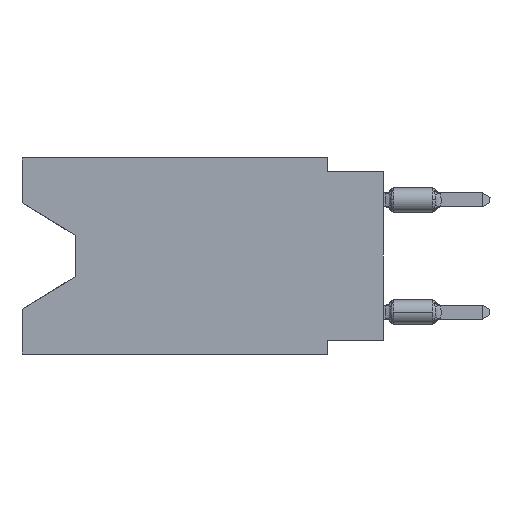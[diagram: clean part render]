
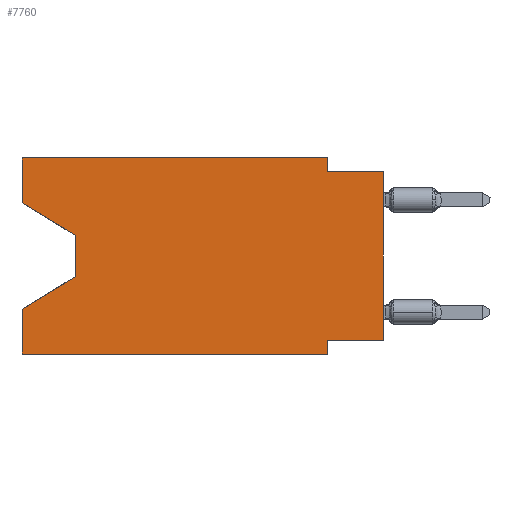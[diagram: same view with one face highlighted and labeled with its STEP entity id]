
A CAD part, left-side view. The second image highlights one B-rep face of the part: STEP entity #7760.
In plain terms, the highlighted planar face has unit normal (-1, 0, 0).
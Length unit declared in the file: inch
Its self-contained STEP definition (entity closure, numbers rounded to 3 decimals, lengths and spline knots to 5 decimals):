
#318 = DIRECTION ( 'NONE',  ( 0., -1., 0. ) ) ;
#1150 = VECTOR ( 'NONE', #9499, 39.37008 ) ;
#1841 = VECTOR ( 'NONE', #16102, 39.37008 ) ;
#2017 = VECTOR ( 'NONE', #31984, 39.37008 ) ;
#2432 = LINE ( 'NONE', #25437, #11160 ) ;
#2998 = LINE ( 'NONE', #15997, #26203 ) ;
#3297 = CARTESIAN_POINT ( 'NONE',  ( 0., 0.645, -0.08025 ) ) ;
#4237 = ORIENTED_EDGE ( 'NONE', *, *, #34123, .F. ) ;
#4421 = LINE ( 'NONE', #14240, #36159 ) ;
#4479 = EDGE_CURVE ( 'NONE', #39658, #11917, #41431, .T. ) ;
#4658 = EDGE_CURVE ( 'NONE', #16934, #17567, #22708, .T. ) ;
#4976 = DIRECTION ( 'NONE',  ( 0., -1., 0. ) ) ;
#7413 = EDGE_CURVE ( 'NONE', #12350, #29813, #33748, .T. ) ;
#7518 = VERTEX_POINT ( 'NONE', #34410 ) ;
#7760 = ADVANCED_FACE ( 'NONE', ( #36956 ), #10735, .F. ) ;
#8228 = VECTOR ( 'NONE', #39567, 39.37008 ) ;
#8532 = VECTOR ( 'NONE', #36527, 39.37008 ) ;
#9341 = CARTESIAN_POINT ( 'NONE',  ( 0., 0., -0.025 ) ) ;
#9465 = CARTESIAN_POINT ( 'NONE',  ( 0., 0.55, -0.138 ) ) ;
#9499 = DIRECTION ( 'NONE',  ( 0., -0.855, -0.519 ) ) ;
#10164 = ORIENTED_EDGE ( 'NONE', *, *, #4479, .F. ) ;
#10735 = PLANE ( 'NONE',  #25814 ) ;
#11044 = VERTEX_POINT ( 'NONE', #17117 ) ;
#11150 = DIRECTION ( 'NONE',  ( 1., 0., 0. ) ) ;
#11160 = VECTOR ( 'NONE', #28229, 39.37008 ) ;
#11300 = ORIENTED_EDGE ( 'NONE', *, *, #36646, .F. ) ;
#11349 = DIRECTION ( 'NONE',  ( 0., 0., -1. ) ) ;
#11610 = VECTOR ( 'NONE', #28250, 39.37008 ) ;
#11917 = VERTEX_POINT ( 'NONE', #25772 ) ;
#12350 = VERTEX_POINT ( 'NONE', #20180 ) ;
#12789 = EDGE_CURVE ( 'NONE', #12350, #17078, #19299, .T. ) ;
#13337 = EDGE_LOOP ( 'NONE', ( #37701, #33000, #29234, #34157, #21272, #28430, #10164, #22071, #40566, #4237, #11300, #14160 ) ) ;
#13786 = LINE ( 'NONE', #23162, #8228 ) ;
#14160 = ORIENTED_EDGE ( 'NONE', *, *, #7413, .F. ) ;
#14240 = CARTESIAN_POINT ( 'NONE',  ( 0., 0., 0. ) ) ;
#14270 = EDGE_CURVE ( 'NONE', #26141, #36155, #41878, .T. ) ;
#14952 = CARTESIAN_POINT ( 'NONE',  ( 0., 0.1, -0.025 ) ) ;
#15997 = CARTESIAN_POINT ( 'NONE',  ( 0., 0.645, -0.35 ) ) ;
#16000 = CARTESIAN_POINT ( 'NONE',  ( 0., 0.55, -0.138 ) ) ;
#16102 = DIRECTION ( 'NONE',  ( 0., 0., 1. ) ) ;
#16518 = VERTEX_POINT ( 'NONE', #24857 ) ;
#16934 = VERTEX_POINT ( 'NONE', #14952 ) ;
#17078 = VERTEX_POINT ( 'NONE', #16000 ) ;
#17117 = CARTESIAN_POINT ( 'NONE',  ( 0., 0.55, -0.212 ) ) ;
#17206 = CARTESIAN_POINT ( 'NONE',  ( 0., 0.645, -0.26975 ) ) ;
#17561 = CARTESIAN_POINT ( 'NONE',  ( 0., 0.645, 0. ) ) ;
#17567 = VERTEX_POINT ( 'NONE', #9341 ) ;
#17666 = CARTESIAN_POINT ( 'NONE',  ( 0., 0.645, -0.35 ) ) ;
#18303 = EDGE_CURVE ( 'NONE', #26141, #7518, #2998, .T. ) ;
#18371 = VECTOR ( 'NONE', #4976, 39.37008 ) ;
#19299 = LINE ( 'NONE', #3297, #1150 ) ;
#19459 = DIRECTION ( 'NONE',  ( 0., 0., -1. ) ) ;
#20180 = CARTESIAN_POINT ( 'NONE',  ( 0., 0.645, -0.08025 ) ) ;
#21272 = ORIENTED_EDGE ( 'NONE', *, *, #18303, .T. ) ;
#22071 = ORIENTED_EDGE ( 'NONE', *, *, #28123, .T. ) ;
#22308 = CARTESIAN_POINT ( 'NONE',  ( 0., 0.645, 0. ) ) ;
#22396 = CARTESIAN_POINT ( 'NONE',  ( 0., 0.1, -0.35 ) ) ;
#22708 = LINE ( 'NONE', #28886, #28621 ) ;
#23162 = CARTESIAN_POINT ( 'NONE',  ( 0., 0.55, -0.212 ) ) ;
#24857 = CARTESIAN_POINT ( 'NONE',  ( 0., 0.1, 0. ) ) ;
#25437 = CARTESIAN_POINT ( 'NONE',  ( 0., 0.1, 0. ) ) ;
#25772 = CARTESIAN_POINT ( 'NONE',  ( 0., 0.1, -0.325 ) ) ;
#25814 = AXIS2_PLACEMENT_3D ( 'NONE', #40529, #11150, #11349 ) ;
#26141 = VERTEX_POINT ( 'NONE', #17666 ) ;
#26200 = LINE ( 'NONE', #22396, #2017 ) ;
#26203 = VECTOR ( 'NONE', #29211, 39.37008 ) ;
#28123 = EDGE_CURVE ( 'NONE', #39658, #17567, #4421, .T. ) ;
#28229 = DIRECTION ( 'NONE',  ( 0., 0., -1. ) ) ;
#28250 = DIRECTION ( 'NONE',  ( 0., 1., 0. ) ) ;
#28430 = ORIENTED_EDGE ( 'NONE', *, *, #38281, .F. ) ;
#28621 = VECTOR ( 'NONE', #318, 39.37008 ) ;
#28886 = CARTESIAN_POINT ( 'NONE',  ( 0., 0., -0.025 ) ) ;
#29211 = DIRECTION ( 'NONE',  ( 0., -1., 0. ) ) ;
#29234 = ORIENTED_EDGE ( 'NONE', *, *, #31005, .T. ) ;
#29813 = VERTEX_POINT ( 'NONE', #30189 ) ;
#29975 = CARTESIAN_POINT ( 'NONE',  ( 0., 0., -0.325 ) ) ;
#30189 = CARTESIAN_POINT ( 'NONE',  ( 0., 0.645, 0. ) ) ;
#31005 = EDGE_CURVE ( 'NONE', #11044, #36155, #13786, .T. ) ;
#31984 = DIRECTION ( 'NONE',  ( 0., 0., -1. ) ) ;
#33000 = ORIENTED_EDGE ( 'NONE', *, *, #36766, .T. ) ;
#33748 = LINE ( 'NONE', #17561, #8532 ) ;
#34123 = EDGE_CURVE ( 'NONE', #16518, #16934, #2432, .T. ) ;
#34157 = ORIENTED_EDGE ( 'NONE', *, *, #14270, .F. ) ;
#34256 = DIRECTION ( 'NONE',  ( 0., 0., 1. ) ) ;
#34410 = CARTESIAN_POINT ( 'NONE',  ( 0., 0.1, -0.35 ) ) ;
#36155 = VERTEX_POINT ( 'NONE', #17206 ) ;
#36159 = VECTOR ( 'NONE', #34256, 39.37008 ) ;
#36527 = DIRECTION ( 'NONE',  ( 0., 0., 1. ) ) ;
#36646 = EDGE_CURVE ( 'NONE', #29813, #16518, #37604, .T. ) ;
#36766 = EDGE_CURVE ( 'NONE', #17078, #11044, #38855, .T. ) ;
#36956 = FACE_OUTER_BOUND ( 'NONE', #13337, .T. ) ;
#37604 = LINE ( 'NONE', #41391, #18371 ) ;
#37701 = ORIENTED_EDGE ( 'NONE', *, *, #12789, .T. ) ;
#38281 = EDGE_CURVE ( 'NONE', #11917, #7518, #26200, .T. ) ;
#38855 = LINE ( 'NONE', #9465, #40016 ) ;
#39567 = DIRECTION ( 'NONE',  ( 0., 0.855, -0.519 ) ) ;
#39658 = VERTEX_POINT ( 'NONE', #29975 ) ;
#40016 = VECTOR ( 'NONE', #19459, 39.37008 ) ;
#40529 = CARTESIAN_POINT ( 'NONE',  ( 0., 0.645, 0. ) ) ;
#40566 = ORIENTED_EDGE ( 'NONE', *, *, #4658, .F. ) ;
#41391 = CARTESIAN_POINT ( 'NONE',  ( 0., 0.645, 0. ) ) ;
#41431 = LINE ( 'NONE', #41644, #11610 ) ;
#41644 = CARTESIAN_POINT ( 'NONE',  ( 0., 0., -0.325 ) ) ;
#41878 = LINE ( 'NONE', #22308, #1841 ) ;
